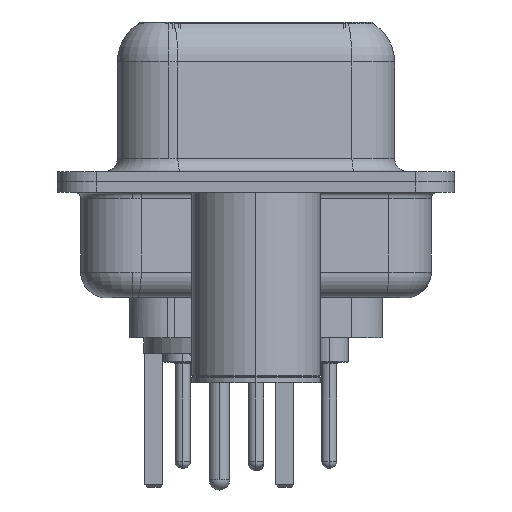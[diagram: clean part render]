
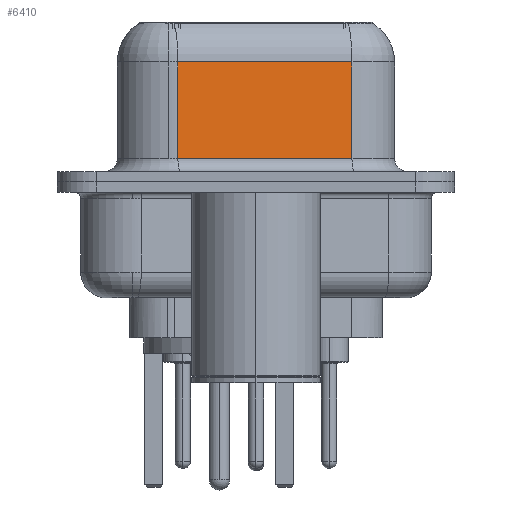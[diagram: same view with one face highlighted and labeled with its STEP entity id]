
A CAD part, left-side view. The second image highlights one B-rep face of the part: STEP entity #6410.
In plain terms, the highlighted planar face has unit normal (-0.985, -0.174, 0).
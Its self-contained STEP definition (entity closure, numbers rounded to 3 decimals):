
#179 = LINE ( 'NONE', #2780, #29307 ) ;
#858 = FACE_OUTER_BOUND ( 'NONE', #29197, .T. ) ;
#2313 = CARTESIAN_POINT ( 'NONE',  ( 5.621, -3.722, 4.65 ) ) ;
#2346 = LINE ( 'NONE', #31039, #12922 ) ;
#2780 = CARTESIAN_POINT ( 'NONE',  ( 5.621, -3.722, 6.4 ) ) ;
#4730 = EDGE_CURVE ( 'NONE', #15168, #31754, #19515, .T. ) ;
#5192 = DIRECTION ( 'NONE',  ( -0.174, 0.985, 0. ) ) ;
#5426 = VERTEX_POINT ( 'NONE', #2313 ) ;
#6410 = ADVANCED_FACE ( 'NONE', ( #858 ), #10838, .F. ) ;
#8425 = DIRECTION ( 'NONE',  ( 0., 0., -1. ) ) ;
#8796 = ORIENTED_EDGE ( 'NONE', *, *, #29705, .T. ) ;
#9483 = ORIENTED_EDGE ( 'NONE', *, *, #24384, .T. ) ;
#10824 = CARTESIAN_POINT ( 'NONE',  ( 5.621, -3.722, 4.65 ) ) ;
#10838 = PLANE ( 'NONE',  #17615 ) ;
#12922 = VECTOR ( 'NONE', #16992, 1000. ) ;
#13408 = EDGE_CURVE ( 'NONE', #5426, #31754, #179, .T. ) ;
#15168 = VERTEX_POINT ( 'NONE', #30124 ) ;
#15504 = VECTOR ( 'NONE', #25917, 1000. ) ;
#16108 = CARTESIAN_POINT ( 'NONE',  ( 5.621, -3.722, 0.9 ) ) ;
#16394 = LINE ( 'NONE', #10824, #15504 ) ;
#16992 = DIRECTION ( 'NONE',  ( 0., 0., -1. ) ) ;
#17615 = AXIS2_PLACEMENT_3D ( 'NONE', #30620, #30497, #5192 ) ;
#19515 = LINE ( 'NONE', #16108, #33206 ) ;
#22196 = CARTESIAN_POINT ( 'NONE',  ( 5.621, -3.722, 0.9 ) ) ;
#24384 = EDGE_CURVE ( 'NONE', #5426, #32179, #16394, .T. ) ;
#25917 = DIRECTION ( 'NONE',  ( -0.174, 0.985, 0. ) ) ;
#29197 = EDGE_LOOP ( 'NONE', ( #33127, #9483, #8796, #29543 ) ) ;
#29307 = VECTOR ( 'NONE', #8425, 1000. ) ;
#29543 = ORIENTED_EDGE ( 'NONE', *, *, #4730, .T. ) ;
#29705 = EDGE_CURVE ( 'NONE', #32179, #15168, #2346, .T. ) ;
#30124 = CARTESIAN_POINT ( 'NONE',  ( 4.43, 3.028, 0.9 ) ) ;
#30497 = DIRECTION ( 'NONE',  ( 0.985, 0.174, 0. ) ) ;
#30620 = CARTESIAN_POINT ( 'NONE',  ( 5.621, -3.722, 6.4 ) ) ;
#31039 = CARTESIAN_POINT ( 'NONE',  ( 4.43, 3.028, 6.4 ) ) ;
#31754 = VERTEX_POINT ( 'NONE', #22196 ) ;
#32179 = VERTEX_POINT ( 'NONE', #32409 ) ;
#32409 = CARTESIAN_POINT ( 'NONE',  ( 4.43, 3.028, 4.65 ) ) ;
#32902 = DIRECTION ( 'NONE',  ( 0.174, -0.985, 0. ) ) ;
#33127 = ORIENTED_EDGE ( 'NONE', *, *, #13408, .F. ) ;
#33206 = VECTOR ( 'NONE', #32902, 1000. ) ;
